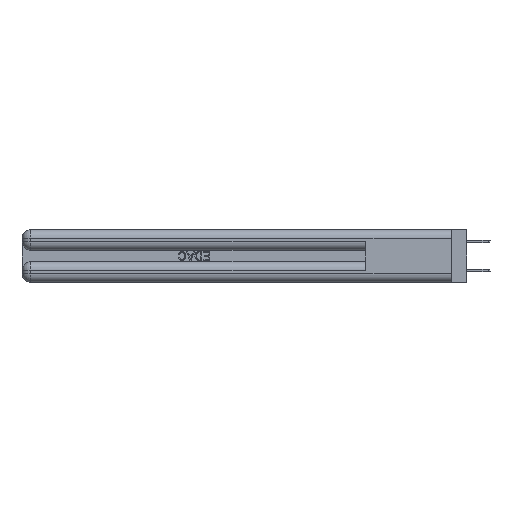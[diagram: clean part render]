
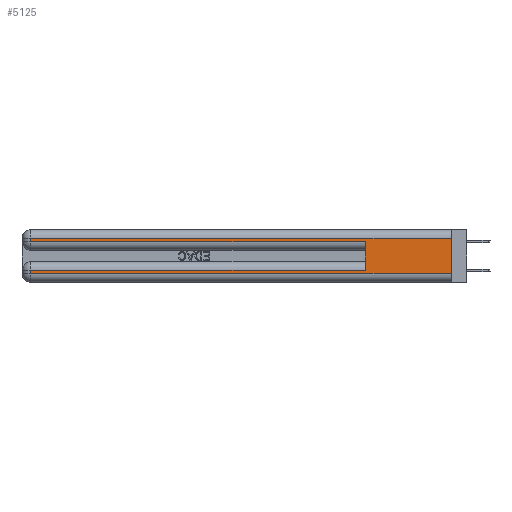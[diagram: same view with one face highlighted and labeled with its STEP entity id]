
A CAD part, left-side view. The second image highlights one B-rep face of the part: STEP entity #5125.
In plain terms, the highlighted planar face has unit normal (-1, 0, 0).
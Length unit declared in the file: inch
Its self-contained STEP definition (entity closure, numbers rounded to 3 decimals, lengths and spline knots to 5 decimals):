
#1413 = AXIS2_PLACEMENT_3D ( 'NONE', #28752, #35117, #16128 ) ;
#1539 = CARTESIAN_POINT ( 'NONE',  ( 0., 0.6, 0.085 ) ) ;
#1593 = CARTESIAN_POINT ( 'NONE',  ( 0., 0., 0.06 ) ) ;
#1605 = CARTESIAN_POINT ( 'NONE',  ( 0., 0., 0.37 ) ) ;
#1959 = CARTESIAN_POINT ( 'NONE',  ( 0., 2.94, 0.285 ) ) ;
#2506 = VECTOR ( 'NONE', #32359, 39.37008 ) ;
#3212 = CARTESIAN_POINT ( 'NONE',  ( 0., 2.94, 0.31 ) ) ;
#3433 = PLANE ( 'NONE',  #1413 ) ;
#4383 = VECTOR ( 'NONE', #17811, 39.37008 ) ;
#4498 = FACE_OUTER_BOUND ( 'NONE', #31062, .T. ) ;
#4623 = VERTEX_POINT ( 'NONE', #1539 ) ;
#4626 = VERTEX_POINT ( 'NONE', #4692 ) ;
#4692 = CARTESIAN_POINT ( 'NONE',  ( 0., 0., 0.06 ) ) ;
#5125 = ADVANCED_FACE ( 'NONE', ( #4498 ), #3433, .F. ) ;
#5897 = EDGE_CURVE ( 'NONE', #4623, #25829, #12342, .T. ) ;
#5947 = ORIENTED_EDGE ( 'NONE', *, *, #28748, .T. ) ;
#6486 = VERTEX_POINT ( 'NONE', #1959 ) ;
#6491 = EDGE_CURVE ( 'NONE', #16202, #8577, #21174, .T. ) ;
#8577 = VERTEX_POINT ( 'NONE', #20201 ) ;
#10312 = ORIENTED_EDGE ( 'NONE', *, *, #40096, .F. ) ;
#10660 = VECTOR ( 'NONE', #20350, 39.37008 ) ;
#10974 = CARTESIAN_POINT ( 'NONE',  ( 0., 2.94, 0.37 ) ) ;
#11143 = ORIENTED_EDGE ( 'NONE', *, *, #12421, .T. ) ;
#12342 = LINE ( 'NONE', #29501, #34639 ) ;
#12421 = EDGE_CURVE ( 'NONE', #6486, #25829, #32871, .T. ) ;
#12581 = VECTOR ( 'NONE', #33249, 39.37008 ) ;
#12684 = VECTOR ( 'NONE', #17435, 39.37008 ) ;
#15754 = DIRECTION ( 'NONE',  ( 0., -1., 0. ) ) ;
#16021 = VECTOR ( 'NONE', #15754, 39.37008 ) ;
#16128 = DIRECTION ( 'NONE',  ( 0., 0., -1. ) ) ;
#16202 = VERTEX_POINT ( 'NONE', #40395 ) ;
#16559 = ORIENTED_EDGE ( 'NONE', *, *, #17360, .T. ) ;
#17360 = EDGE_CURVE ( 'NONE', #24367, #6486, #20031, .T. ) ;
#17435 = DIRECTION ( 'NONE',  ( 0., -1., 0. ) ) ;
#17468 = ORIENTED_EDGE ( 'NONE', *, *, #6491, .T. ) ;
#17811 = DIRECTION ( 'NONE',  ( 0., 0., -1. ) ) ;
#18786 = CARTESIAN_POINT ( 'NONE',  ( 0., 0., 0.285 ) ) ;
#20031 = LINE ( 'NONE', #10974, #10660 ) ;
#20079 = DIRECTION ( 'NONE',  ( 0., 0., 1. ) ) ;
#20201 = CARTESIAN_POINT ( 'NONE',  ( 0., 2.94, 0.06 ) ) ;
#20350 = DIRECTION ( 'NONE',  ( 0., 0., -1. ) ) ;
#21116 = CARTESIAN_POINT ( 'NONE',  ( 0., 0., 0.31 ) ) ;
#21174 = LINE ( 'NONE', #33620, #4383 ) ;
#21404 = CARTESIAN_POINT ( 'NONE',  ( 0., 0.6, 0.285 ) ) ;
#24064 = EDGE_CURVE ( 'NONE', #8577, #4626, #28544, .T. ) ;
#24096 = DIRECTION ( 'NONE',  ( 0., 1., 0. ) ) ;
#24177 = EDGE_CURVE ( 'NONE', #4623, #16202, #25576, .T. ) ;
#24367 = VERTEX_POINT ( 'NONE', #3212 ) ;
#24563 = VECTOR ( 'NONE', #24096, 39.37008 ) ;
#25576 = LINE ( 'NONE', #40180, #24563 ) ;
#25829 = VERTEX_POINT ( 'NONE', #21404 ) ;
#27353 = ORIENTED_EDGE ( 'NONE', *, *, #24064, .T. ) ;
#28544 = LINE ( 'NONE', #1593, #12684 ) ;
#28722 = LINE ( 'NONE', #29161, #2506 ) ;
#28748 = EDGE_CURVE ( 'NONE', #30349, #24367, #28722, .T. ) ;
#28752 = CARTESIAN_POINT ( 'NONE',  ( 0., 0., 0.37 ) ) ;
#28766 = ORIENTED_EDGE ( 'NONE', *, *, #24177, .T. ) ;
#29161 = CARTESIAN_POINT ( 'NONE',  ( 0., 0., 0.31 ) ) ;
#29501 = CARTESIAN_POINT ( 'NONE',  ( 0., 0.6, 0.145 ) ) ;
#30349 = VERTEX_POINT ( 'NONE', #21116 ) ;
#31062 = EDGE_LOOP ( 'NONE', ( #10312, #5947, #16559, #11143, #38184, #28766, #17468, #27353 ) ) ;
#32359 = DIRECTION ( 'NONE',  ( 0., 1., 0. ) ) ;
#32871 = LINE ( 'NONE', #18786, #16021 ) ;
#33249 = DIRECTION ( 'NONE',  ( 0., 0., -1. ) ) ;
#33620 = CARTESIAN_POINT ( 'NONE',  ( 0., 2.94, 0.37 ) ) ;
#34639 = VECTOR ( 'NONE', #20079, 39.37008 ) ;
#35117 = DIRECTION ( 'NONE',  ( 1., 0., 0. ) ) ;
#37837 = LINE ( 'NONE', #1605, #12581 ) ;
#38184 = ORIENTED_EDGE ( 'NONE', *, *, #5897, .F. ) ;
#40096 = EDGE_CURVE ( 'NONE', #30349, #4626, #37837, .T. ) ;
#40180 = CARTESIAN_POINT ( 'NONE',  ( 0., 0., 0.085 ) ) ;
#40395 = CARTESIAN_POINT ( 'NONE',  ( 0., 2.94, 0.085 ) ) ;
